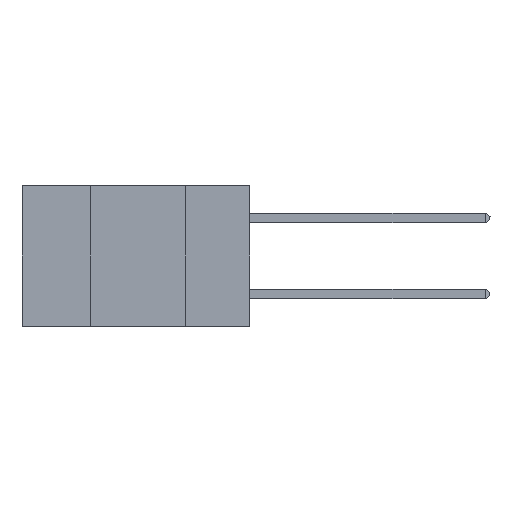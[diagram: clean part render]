
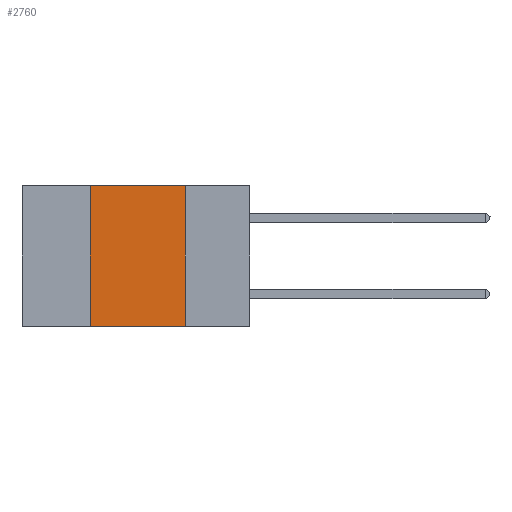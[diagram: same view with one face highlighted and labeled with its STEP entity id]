
A CAD part, left-side view. The second image highlights one B-rep face of the part: STEP entity #2760.
In plain terms, the highlighted planar face has unit normal (-1, 0, 0).
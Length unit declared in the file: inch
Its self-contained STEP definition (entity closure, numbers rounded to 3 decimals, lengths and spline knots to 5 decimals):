
#257 = ORIENTED_EDGE ( 'NONE', *, *, #6791, .F. ) ;
#1560 = ORIENTED_EDGE ( 'NONE', *, *, #23334, .T. ) ;
#2321 = VERTEX_POINT ( 'NONE', #32254 ) ;
#2760 = ADVANCED_FACE ( 'NONE', ( #7467 ), #26319, .F. ) ;
#3424 = AXIS2_PLACEMENT_3D ( 'NONE', #29368, #26141, #7277 ) ;
#6727 = VECTOR ( 'NONE', #24886, 39.37008 ) ;
#6791 = EDGE_CURVE ( 'NONE', #26971, #14135, #29911, .T. ) ;
#7277 = DIRECTION ( 'NONE',  ( 0., 0., -1. ) ) ;
#7467 = FACE_OUTER_BOUND ( 'NONE', #18212, .T. ) ;
#7948 = ORIENTED_EDGE ( 'NONE', *, *, #9041, .F. ) ;
#8198 = CARTESIAN_POINT ( 'NONE',  ( 0., 0.6, 0. ) ) ;
#9041 = EDGE_CURVE ( 'NONE', #2321, #26971, #32412, .T. ) ;
#12453 = CARTESIAN_POINT ( 'NONE',  ( 0., 0.17, 0. ) ) ;
#14135 = VERTEX_POINT ( 'NONE', #34280 ) ;
#17695 = LINE ( 'NONE', #12453, #34418 ) ;
#18212 = EDGE_LOOP ( 'NONE', ( #19361, #257, #7948, #1560 ) ) ;
#19361 = ORIENTED_EDGE ( 'NONE', *, *, #24913, .F. ) ;
#20684 = VERTEX_POINT ( 'NONE', #32191 ) ;
#20783 = CARTESIAN_POINT ( 'NONE',  ( 0., 0.6, -0.37 ) ) ;
#22820 = CARTESIAN_POINT ( 'NONE',  ( 0., 0.42, 0. ) ) ;
#23158 = VECTOR ( 'NONE', #23507, 39.37008 ) ;
#23334 = EDGE_CURVE ( 'NONE', #2321, #20684, #27057, .T. ) ;
#23507 = DIRECTION ( 'NONE',  ( 0., 0., 1. ) ) ;
#24033 = CARTESIAN_POINT ( 'NONE',  ( 0., 0.42, 0. ) ) ;
#24886 = DIRECTION ( 'NONE',  ( 0., -1., 0. ) ) ;
#24913 = EDGE_CURVE ( 'NONE', #14135, #20684, #17695, .T. ) ;
#26141 = DIRECTION ( 'NONE',  ( 1., 0., 0. ) ) ;
#26319 = PLANE ( 'NONE',  #3424 ) ;
#26971 = VERTEX_POINT ( 'NONE', #22820 ) ;
#27057 = LINE ( 'NONE', #20783, #31497 ) ;
#29368 = CARTESIAN_POINT ( 'NONE',  ( 0., 0.6, 0. ) ) ;
#29381 = DIRECTION ( 'NONE',  ( 0., -1., 0. ) ) ;
#29911 = LINE ( 'NONE', #8198, #6727 ) ;
#31497 = VECTOR ( 'NONE', #29381, 39.37008 ) ;
#32191 = CARTESIAN_POINT ( 'NONE',  ( 0., 0.17, -0.37 ) ) ;
#32254 = CARTESIAN_POINT ( 'NONE',  ( 0., 0.42, -0.37 ) ) ;
#32412 = LINE ( 'NONE', #24033, #23158 ) ;
#33643 = DIRECTION ( 'NONE',  ( 0., 0., -1. ) ) ;
#34280 = CARTESIAN_POINT ( 'NONE',  ( 0., 0.17, 0. ) ) ;
#34418 = VECTOR ( 'NONE', #33643, 39.37008 ) ;
